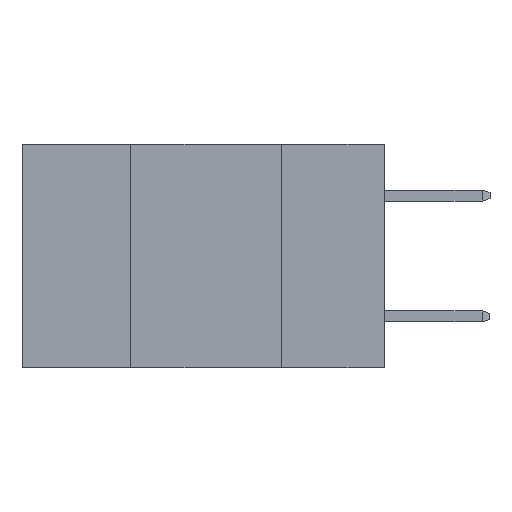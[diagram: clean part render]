
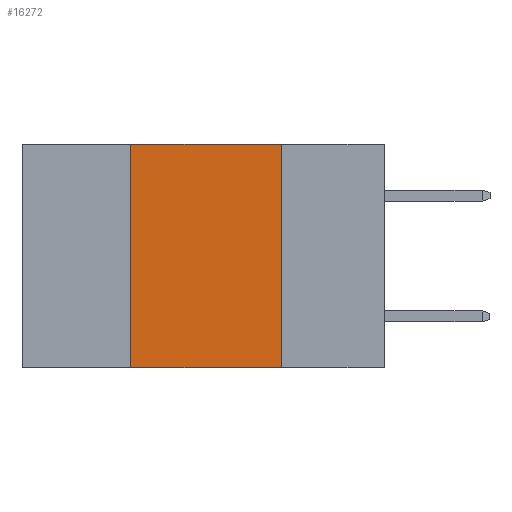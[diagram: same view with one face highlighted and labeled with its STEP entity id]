
A CAD part, left-side view. The second image highlights one B-rep face of the part: STEP entity #16272.
In plain terms, the highlighted planar face has unit normal (-1, 0, 0).
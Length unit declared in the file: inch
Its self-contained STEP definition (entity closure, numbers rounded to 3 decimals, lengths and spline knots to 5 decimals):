
#692 = ORIENTED_EDGE ( 'NONE', *, *, #15297, .T. ) ;
#1796 = CARTESIAN_POINT ( 'NONE',  ( 0., 0.17, -0.37 ) ) ;
#1973 = VECTOR ( 'NONE', #7731, 39.37008 ) ;
#3401 = ORIENTED_EDGE ( 'NONE', *, *, #22410, .F. ) ;
#3559 = CARTESIAN_POINT ( 'NONE',  ( 0., 0.17, 0. ) ) ;
#5508 = CARTESIAN_POINT ( 'NONE',  ( 0., 0.42, 0. ) ) ;
#5934 = EDGE_LOOP ( 'NONE', ( #3401, #9908, #15196, #692 ) ) ;
#5983 = PLANE ( 'NONE',  #14265 ) ;
#6524 = LINE ( 'NONE', #13234, #12977 ) ;
#7731 = DIRECTION ( 'NONE',  ( 0., 0., 1. ) ) ;
#9908 = ORIENTED_EDGE ( 'NONE', *, *, #15256, .F. ) ;
#10376 = DIRECTION ( 'NONE',  ( 1., 0., 0. ) ) ;
#10409 = VERTEX_POINT ( 'NONE', #1796 ) ;
#11536 = CARTESIAN_POINT ( 'NONE',  ( 0., 0.42, 0. ) ) ;
#11866 = LINE ( 'NONE', #14723, #27305 ) ;
#12977 = VECTOR ( 'NONE', #15321, 39.37008 ) ;
#13234 = CARTESIAN_POINT ( 'NONE',  ( 0., 0.6, -0.37 ) ) ;
#14265 = AXIS2_PLACEMENT_3D ( 'NONE', #20943, #10376, #25173 ) ;
#14723 = CARTESIAN_POINT ( 'NONE',  ( 0., 0.17, 0. ) ) ;
#15196 = ORIENTED_EDGE ( 'NONE', *, *, #26879, .F. ) ;
#15256 = EDGE_CURVE ( 'NONE', #26742, #25166, #19248, .T. ) ;
#15297 = EDGE_CURVE ( 'NONE', #19462, #10409, #6524, .T. ) ;
#15321 = DIRECTION ( 'NONE',  ( 0., -1., 0. ) ) ;
#16210 = FACE_OUTER_BOUND ( 'NONE', #5934, .T. ) ;
#16272 = ADVANCED_FACE ( 'NONE', ( #16210 ), #5983, .F. ) ;
#16847 = DIRECTION ( 'NONE',  ( 0., 0., -1. ) ) ;
#18570 = VECTOR ( 'NONE', #25740, 39.37008 ) ;
#19120 = LINE ( 'NONE', #5508, #1973 ) ;
#19248 = LINE ( 'NONE', #19427, #18570 ) ;
#19427 = CARTESIAN_POINT ( 'NONE',  ( 0., 0.6, 0. ) ) ;
#19462 = VERTEX_POINT ( 'NONE', #26353 ) ;
#20943 = CARTESIAN_POINT ( 'NONE',  ( 0., 0.6, 0. ) ) ;
#22410 = EDGE_CURVE ( 'NONE', #25166, #10409, #11866, .T. ) ;
#25166 = VERTEX_POINT ( 'NONE', #3559 ) ;
#25173 = DIRECTION ( 'NONE',  ( 0., 0., -1. ) ) ;
#25740 = DIRECTION ( 'NONE',  ( 0., -1., 0. ) ) ;
#26353 = CARTESIAN_POINT ( 'NONE',  ( 0., 0.42, -0.37 ) ) ;
#26742 = VERTEX_POINT ( 'NONE', #11536 ) ;
#26879 = EDGE_CURVE ( 'NONE', #19462, #26742, #19120, .T. ) ;
#27305 = VECTOR ( 'NONE', #16847, 39.37008 ) ;
